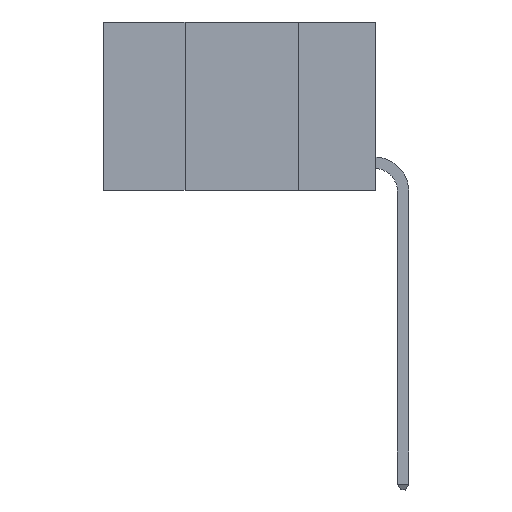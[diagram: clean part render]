
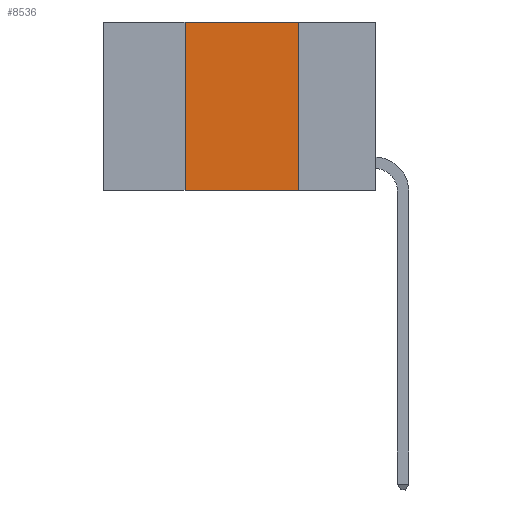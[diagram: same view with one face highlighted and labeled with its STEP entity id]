
A CAD part, left-side view. The second image highlights one B-rep face of the part: STEP entity #8536.
In plain terms, the highlighted planar face has unit normal (-1, 0, 0).
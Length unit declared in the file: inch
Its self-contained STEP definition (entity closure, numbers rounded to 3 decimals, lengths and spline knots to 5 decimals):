
#828 = DIRECTION ( 'NONE',  ( 0., 0., -1. ) ) ;
#1055 = EDGE_CURVE ( 'NONE', #19868, #24635, #7691, .T. ) ;
#1265 = CARTESIAN_POINT ( 'NONE',  ( 0., 0.42, 0. ) ) ;
#3064 = LINE ( 'NONE', #8497, #18045 ) ;
#3324 = AXIS2_PLACEMENT_3D ( 'NONE', #24236, #12550, #828 ) ;
#5602 = EDGE_CURVE ( 'NONE', #8347, #24635, #3064, .T. ) ;
#5740 = LINE ( 'NONE', #20646, #15455 ) ;
#6624 = VERTEX_POINT ( 'NONE', #25306 ) ;
#7654 = EDGE_CURVE ( 'NONE', #6624, #19868, #5740, .T. ) ;
#7691 = LINE ( 'NONE', #14005, #18056 ) ;
#8347 = VERTEX_POINT ( 'NONE', #21695 ) ;
#8497 = CARTESIAN_POINT ( 'NONE',  ( 0., 0.6, -0.37 ) ) ;
#8512 = EDGE_LOOP ( 'NONE', ( #15606, #15728, #16442, #16510 ) ) ;
#8536 = ADVANCED_FACE ( 'NONE', ( #10845 ), #16403, .F. ) ;
#8704 = EDGE_CURVE ( 'NONE', #8347, #6624, #17564, .T. ) ;
#9917 = CARTESIAN_POINT ( 'NONE',  ( 0., 0.17, -0.37 ) ) ;
#10845 = FACE_OUTER_BOUND ( 'NONE', #8512, .T. ) ;
#12550 = DIRECTION ( 'NONE',  ( 1., 0., 0. ) ) ;
#14005 = CARTESIAN_POINT ( 'NONE',  ( 0., 0.17, 0. ) ) ;
#14405 = CARTESIAN_POINT ( 'NONE',  ( 0., 0.17, 0. ) ) ;
#15455 = VECTOR ( 'NONE', #22639, 39.37008 ) ;
#15606 = ORIENTED_EDGE ( 'NONE', *, *, #1055, .F. ) ;
#15728 = ORIENTED_EDGE ( 'NONE', *, *, #7654, .F. ) ;
#16403 = PLANE ( 'NONE',  #3324 ) ;
#16442 = ORIENTED_EDGE ( 'NONE', *, *, #8704, .F. ) ;
#16510 = ORIENTED_EDGE ( 'NONE', *, *, #5602, .T. ) ;
#17564 = LINE ( 'NONE', #1265, #21519 ) ;
#18045 = VECTOR ( 'NONE', #24078, 39.37008 ) ;
#18056 = VECTOR ( 'NONE', #19354, 39.37008 ) ;
#18866 = DIRECTION ( 'NONE',  ( 0., 0., 1. ) ) ;
#19354 = DIRECTION ( 'NONE',  ( 0., 0., -1. ) ) ;
#19868 = VERTEX_POINT ( 'NONE', #14405 ) ;
#20646 = CARTESIAN_POINT ( 'NONE',  ( 0., 0.6, 0. ) ) ;
#21519 = VECTOR ( 'NONE', #18866, 39.37008 ) ;
#21695 = CARTESIAN_POINT ( 'NONE',  ( 0., 0.42, -0.37 ) ) ;
#22639 = DIRECTION ( 'NONE',  ( 0., -1., 0. ) ) ;
#24078 = DIRECTION ( 'NONE',  ( 0., -1., 0. ) ) ;
#24236 = CARTESIAN_POINT ( 'NONE',  ( 0., 0.6, 0. ) ) ;
#24635 = VERTEX_POINT ( 'NONE', #9917 ) ;
#25306 = CARTESIAN_POINT ( 'NONE',  ( 0., 0.42, 0. ) ) ;
